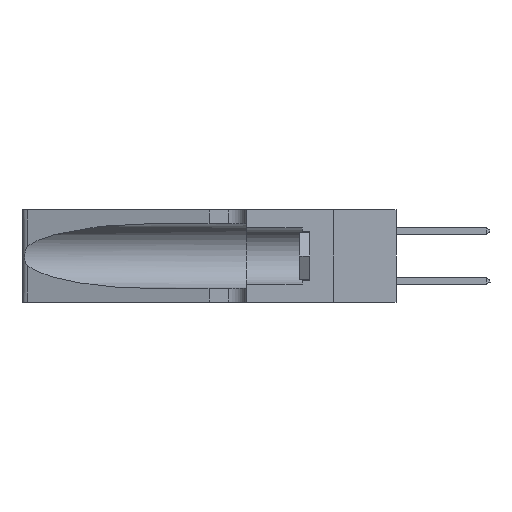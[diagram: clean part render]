
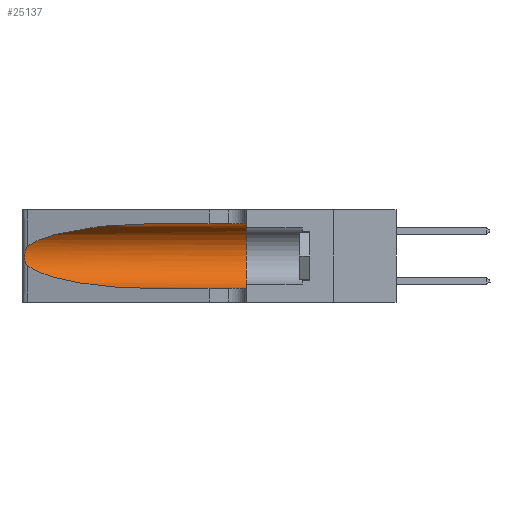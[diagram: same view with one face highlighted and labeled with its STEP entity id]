
A CAD part, left-side view. The second image highlights one B-rep face of the part: STEP entity #25137.
In plain terms, the highlighted cylindrical face has radius 3.308 mm (diameter 6.617 mm), a partial arc.
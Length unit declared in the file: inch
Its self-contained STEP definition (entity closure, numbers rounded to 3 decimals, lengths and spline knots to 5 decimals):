
#3 = DIRECTION ( 'NONE',  ( 0., -1., 0. ) ) ;
#770 = CARTESIAN_POINT ( 'NONE',  ( 0.18966, 0.96281, 0.31525 ) ) ;
#1464 = CARTESIAN_POINT ( 'NONE',  ( 0.1305, 0.35, 0.185 ) ) ;
#1866 = EDGE_CURVE ( 'NONE', #19878, #18407, #26784, .T. ) ;
#2131 = CARTESIAN_POINT ( 'NONE',  ( 0.25555, 1.22994, 0.2215 ) ) ;
#2213 = CARTESIAN_POINT ( 'NONE',  ( 0.25856, 1.23593, 0.16098 ) ) ;
#2754 = CYLINDRICAL_SURFACE ( 'NONE', #9277, 0.13025 ) ;
#2889 = CARTESIAN_POINT ( 'NONE',  ( 0.2373, 1.15595, 0.28018 ) ) ;
#3506 = EDGE_CURVE ( 'NONE', #6347, #26787, #21863, .T. ) ;
#3661 = DIRECTION ( 'NONE',  ( 0., 0., 1. ) ) ;
#4095 = CARTESIAN_POINT ( 'NONE',  ( 0.26075, 1.23896, 0.178 ) ) ;
#4459 = CARTESIAN_POINT ( 'NONE',  ( 0.25639, 1.23186, 0.15144 ) ) ;
#5884 = DIRECTION ( 'NONE',  ( 0., -1., 0. ) ) ;
#6347 = VERTEX_POINT ( 'NONE', #24589 ) ;
#6499 = ORIENTED_EDGE ( 'NONE', *, *, #16035, .T. ) ;
#6611 = CARTESIAN_POINT ( 'NONE',  ( 0.25487, 1.22718, 0.14631 ) ) ;
#6762 = B_SPLINE_CURVE_WITH_KNOTS ( 'NONE', 3,
 ( #21577, #2131, #8702, #23818, #10890, #25905, #13068, #4095, #15256, #2213, #17426, #4459, #19606, #6611 ),
 .UNSPECIFIED., .F., .F.,
 ( 4, 2, 2, 2, 2, 2, 4 ),
 ( 0., 0.00027, 0.00053, 0.00107, 0.0016, 0.00187, 0.00214 ),
 .UNSPECIFIED. ) ;
#7206 = CARTESIAN_POINT ( 'NONE',  ( 0.1305, 0.35, 0.05475 ) ) ;
#7371 = CARTESIAN_POINT ( 'NONE',  ( 0.25487, 1.22718, 0.22369 ) ) ;
#8344 = CARTESIAN_POINT ( 'NONE',  ( 0.18966, 0.96281, 0.05475 ) ) ;
#8393 = DIRECTION ( 'NONE',  ( 0., -1., 0. ) ) ;
#8526 = EDGE_CURVE ( 'NONE', #18407, #6347, #6762, .T. ) ;
#8702 = CARTESIAN_POINT ( 'NONE',  ( 0.25639, 1.23184, 0.21858 ) ) ;
#9277 = AXIS2_PLACEMENT_3D ( 'NONE', #12411, #5884, #27427 ) ;
#9372 = CARTESIAN_POINT ( 'NONE',  ( 0.1305, 0.72297, 0.05475 ) ) ;
#9665 = ORIENTED_EDGE ( 'NONE', *, *, #19796, .F. ) ;
#9934 = CARTESIAN_POINT ( 'NONE',  ( 0.25487, 1.22718, 0.22369 ) ) ;
#10172 = VECTOR ( 'NONE', #3, 39.37008 ) ;
#10514 = CARTESIAN_POINT ( 'NONE',  ( 0.1305, 0.72297, 0.31525 ) ) ;
#10596 = CARTESIAN_POINT ( 'NONE',  ( 0.1305, 1.61858, 0.31525 ) ) ;
#10890 = CARTESIAN_POINT ( 'NONE',  ( 0.25854, 1.2359, 0.20912 ) ) ;
#12411 = CARTESIAN_POINT ( 'NONE',  ( 0.1305, 1.61858, 0.185 ) ) ;
#12416 = CARTESIAN_POINT ( 'NONE',  ( 0.1305, 0.35, 0.31525 ) ) ;
#12720 = CARTESIAN_POINT ( 'NONE',  ( 0.25487, 1.22718, 0.14631 ) ) ;
#13068 = CARTESIAN_POINT ( 'NONE',  ( 0.26075, 1.23896, 0.19203 ) ) ;
#14011 = ORIENTED_EDGE ( 'NONE', *, *, #3506, .T. ) ;
#14331 = FACE_OUTER_BOUND ( 'NONE', #21260, .T. ) ;
#15256 = CARTESIAN_POINT ( 'NONE',  ( 0.26017, 1.23833, 0.17102 ) ) ;
#16035 = EDGE_CURVE ( 'NONE', #26787, #23412, #21666, .T. ) ;
#16687 = DIRECTION ( 'NONE',  ( 0., 1., 0. ) ) ;
#16812 = VECTOR ( 'NONE', #8393, 39.37008 ) ;
#17426 = CARTESIAN_POINT ( 'NONE',  ( 0.25789, 1.23486, 0.15765 ) ) ;
#18407 = VERTEX_POINT ( 'NONE', #9934 ) ;
#18597 = EDGE_CURVE ( 'NONE', #19878, #27062, #25485, .T. ) ;
#18744 = AXIS2_PLACEMENT_3D ( 'NONE', #1464, #16687, #3661 ) ;
#19606 = CARTESIAN_POINT ( 'NONE',  ( 0.25555, 1.22993, 0.14849 ) ) ;
#19796 = EDGE_CURVE ( 'NONE', #27062, #23412, #23781, .T. ) ;
#19878 = VERTEX_POINT ( 'NONE', #10514 ) ;
#20352 = CARTESIAN_POINT ( 'NONE',  ( 0.1305, 0.72297, 0.31525 ) ) ;
#21260 = EDGE_LOOP ( 'NONE', ( #22542, #26986, #14011, #6499, #9665, #26895 ) ) ;
#21577 = CARTESIAN_POINT ( 'NONE',  ( 0.25487, 1.22718, 0.22369 ) ) ;
#21666 = LINE ( 'NONE', #23833, #10172 ) ;
#21863 =( BOUNDED_CURVE ( )  B_SPLINE_CURVE ( 3, ( #12720, #27615, #8344, #27715 ),
 .UNSPECIFIED., .F., .T. ) 
 B_SPLINE_CURVE_WITH_KNOTS ( ( 4, 4 ),
 ( 3.44316, 4.71239 ),
 .UNSPECIFIED. ) 
 CURVE ( )  GEOMETRIC_REPRESENTATION_ITEM ( )  RATIONAL_B_SPLINE_CURVE ( ( 1., 0.87, 0.87, 1. ) ) 
 REPRESENTATION_ITEM ( '' )  );
#22542 = ORIENTED_EDGE ( 'NONE', *, *, #1866, .T. ) ;
#23412 = VERTEX_POINT ( 'NONE', #7206 ) ;
#23781 = CIRCLE ( 'NONE', #18744, 0.13025 ) ;
#23818 = CARTESIAN_POINT ( 'NONE',  ( 0.25787, 1.23484, 0.2124 ) ) ;
#23833 = CARTESIAN_POINT ( 'NONE',  ( 0.1305, 1.61858, 0.05475 ) ) ;
#24589 = CARTESIAN_POINT ( 'NONE',  ( 0.25487, 1.22718, 0.14631 ) ) ;
#25137 = ADVANCED_FACE ( 'NONE', ( #14331 ), #2754, .F. ) ;
#25485 = LINE ( 'NONE', #10596, #16812 ) ;
#25905 = CARTESIAN_POINT ( 'NONE',  ( 0.26018, 1.23835, 0.19895 ) ) ;
#26784 =( BOUNDED_CURVE ( )  B_SPLINE_CURVE ( 3, ( #20352, #770, #2889, #7371 ),
 .UNSPECIFIED., .F., .T. ) 
 B_SPLINE_CURVE_WITH_KNOTS ( ( 4, 4 ),
 ( 1.5708, 2.84003 ),
 .UNSPECIFIED. ) 
 CURVE ( )  GEOMETRIC_REPRESENTATION_ITEM ( )  RATIONAL_B_SPLINE_CURVE ( ( 1., 0.87, 0.87, 1. ) ) 
 REPRESENTATION_ITEM ( '' )  );
#26787 = VERTEX_POINT ( 'NONE', #9372 ) ;
#26895 = ORIENTED_EDGE ( 'NONE', *, *, #18597, .F. ) ;
#26986 = ORIENTED_EDGE ( 'NONE', *, *, #8526, .T. ) ;
#27062 = VERTEX_POINT ( 'NONE', #12416 ) ;
#27427 = DIRECTION ( 'NONE',  ( 0., 0., -1. ) ) ;
#27615 = CARTESIAN_POINT ( 'NONE',  ( 0.2373, 1.15595, 0.08982 ) ) ;
#27715 = CARTESIAN_POINT ( 'NONE',  ( 0.1305, 0.72297, 0.05475 ) ) ;
